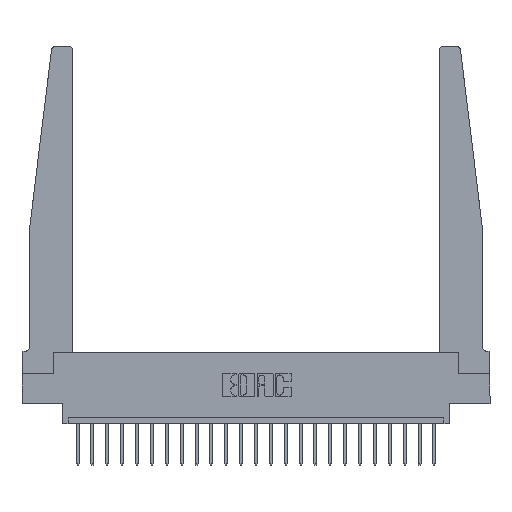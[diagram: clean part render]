
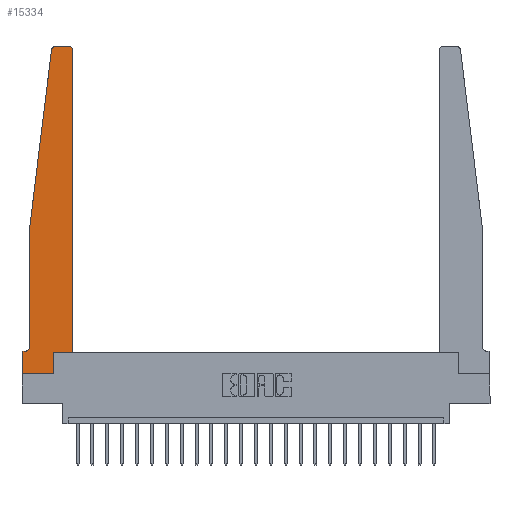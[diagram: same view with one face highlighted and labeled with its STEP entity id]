
A CAD part, top view. The second image highlights one B-rep face of the part: STEP entity #15334.
In plain terms, the highlighted planar face has unit normal (0, 0, 1).
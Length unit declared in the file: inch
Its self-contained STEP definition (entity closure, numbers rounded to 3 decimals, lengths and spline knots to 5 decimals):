
#33 = ORIENTED_EDGE ( 'NONE', *, *, #2046, .T. ) ;
#178 = VECTOR ( 'NONE', #5437, 39.37008 ) ;
#296 = EDGE_CURVE ( 'NONE', #17485, #15107, #15571, .T. ) ;
#578 = VERTEX_POINT ( 'NONE', #1605 ) ;
#906 = CARTESIAN_POINT ( 'NONE',  ( 0., 0.1875, 0.37 ) ) ;
#1040 = VECTOR ( 'NONE', #8068, 39.37008 ) ;
#1192 = CARTESIAN_POINT ( 'NONE',  ( 0.065, 1.25, 0.37 ) ) ;
#1251 = CARTESIAN_POINT ( 'NONE',  ( 0.25, 2.75, 0.37 ) ) ;
#1531 = CARTESIAN_POINT ( 'NONE',  ( 0., 0.1875, 0.37 ) ) ;
#1605 = CARTESIAN_POINT ( 'NONE',  ( 0.015, 0.1875, 0.37 ) ) ;
#2046 = EDGE_CURVE ( 'NONE', #578, #8622, #7884, .T. ) ;
#2065 = CARTESIAN_POINT ( 'NONE',  ( 0., 0., 0.37 ) ) ;
#2200 = DIRECTION ( 'NONE',  ( 1., 0., 0. ) ) ;
#2301 = CARTESIAN_POINT ( 'NONE',  ( 0.425, 0.18, 0.37 ) ) ;
#2494 = LINE ( 'NONE', #1192, #17571 ) ;
#3321 = DIRECTION ( 'NONE',  ( 1., 0., 0. ) ) ;
#3685 = LINE ( 'NONE', #8054, #11895 ) ;
#3726 = VERTEX_POINT ( 'NONE', #7447 ) ;
#3820 = ORIENTED_EDGE ( 'NONE', *, *, #14248, .T. ) ;
#4099 = EDGE_CURVE ( 'NONE', #8622, #10475, #9236, .T. ) ;
#4494 = VECTOR ( 'NONE', #9052, 39.37008 ) ;
#4500 = VECTOR ( 'NONE', #11226, 39.37008 ) ;
#5191 = DIRECTION ( 'NONE',  ( -1., 0., 0. ) ) ;
#5437 = DIRECTION ( 'NONE',  ( 1., 0., 0. ) ) ;
#5623 = LINE ( 'NONE', #1251, #7583 ) ;
#6602 = DIRECTION ( 'NONE',  ( 0., -1., 0. ) ) ;
#6870 = CARTESIAN_POINT ( 'NONE',  ( 0.27653, 2.72, 0.37 ) ) ;
#7027 = DIRECTION ( 'NONE',  ( 0., 0., 1. ) ) ;
#7152 = CIRCLE ( 'NONE', #14906, 0.03 ) ;
#7227 = AXIS2_PLACEMENT_3D ( 'NONE', #16472, #20184, #21952 ) ;
#7410 = ORIENTED_EDGE ( 'NONE', *, *, #16165, .T. ) ;
#7447 = CARTESIAN_POINT ( 'NONE',  ( 0.395, 2.75, 0.37 ) ) ;
#7566 = EDGE_CURVE ( 'NONE', #19655, #578, #7614, .T. ) ;
#7583 = VECTOR ( 'NONE', #5191, 39.37008 ) ;
#7614 = CIRCLE ( 'NONE', #7227, 0.05 ) ;
#7641 = AXIS2_PLACEMENT_3D ( 'NONE', #1531, #13812, #3321 ) ;
#7884 = LINE ( 'NONE', #9121, #17400 ) ;
#7987 = CIRCLE ( 'NONE', #13327, 0.03 ) ;
#8054 = CARTESIAN_POINT ( 'NONE',  ( 0.425, 0.18, 0.37 ) ) ;
#8068 = DIRECTION ( 'NONE',  ( -0.122, -0.992, 0. ) ) ;
#8076 = ORIENTED_EDGE ( 'NONE', *, *, #4099, .T. ) ;
#8575 = VERTEX_POINT ( 'NONE', #14924 ) ;
#8622 = VERTEX_POINT ( 'NONE', #906 ) ;
#9052 = DIRECTION ( 'NONE',  ( 0., -1., 0. ) ) ;
#9121 = CARTESIAN_POINT ( 'NONE',  ( 0.065, 0.1875, 0.37 ) ) ;
#9236 = LINE ( 'NONE', #2065, #4494 ) ;
#9386 = CARTESIAN_POINT ( 'NONE',  ( 0., 0., 0.37 ) ) ;
#9550 = CARTESIAN_POINT ( 'NONE',  ( 0.065, 0.2375, 0.37 ) ) ;
#9798 = CARTESIAN_POINT ( 'NONE',  ( 0.2605, 0.18, 0.37 ) ) ;
#9815 = CARTESIAN_POINT ( 'NONE',  ( 0.065, 1.25, 0.37 ) ) ;
#10367 = ORIENTED_EDGE ( 'NONE', *, *, #19819, .T. ) ;
#10457 = EDGE_LOOP ( 'NONE', ( #3820, #7410, #16579, #10367, #12165, #33, #8076, #15566, #21629, #22363, #20097, #19935 ) ) ;
#10475 = VERTEX_POINT ( 'NONE', #9386 ) ;
#10541 = EDGE_CURVE ( 'NONE', #21972, #19826, #13118, .T. ) ;
#10575 = CARTESIAN_POINT ( 'NONE',  ( 0., 0., 0.37 ) ) ;
#11226 = DIRECTION ( 'NONE',  ( 0., 1., 0. ) ) ;
#11419 = EDGE_CURVE ( 'NONE', #10475, #14870, #13098, .T. ) ;
#11895 = VECTOR ( 'NONE', #14939, 39.37008 ) ;
#12165 = ORIENTED_EDGE ( 'NONE', *, *, #7566, .T. ) ;
#12744 = LINE ( 'NONE', #9798, #4500 ) ;
#12791 = EDGE_CURVE ( 'NONE', #14870, #17485, #12744, .T. ) ;
#13098 = LINE ( 'NONE', #10575, #178 ) ;
#13118 = LINE ( 'NONE', #9815, #1040 ) ;
#13327 = AXIS2_PLACEMENT_3D ( 'NONE', #6870, #13493, #19040 ) ;
#13493 = DIRECTION ( 'NONE',  ( 0., 0., 1. ) ) ;
#13812 = DIRECTION ( 'NONE',  ( 0., 0., 1. ) ) ;
#14248 = EDGE_CURVE ( 'NONE', #3726, #8575, #5623, .T. ) ;
#14870 = VERTEX_POINT ( 'NONE', #20574 ) ;
#14906 = AXIS2_PLACEMENT_3D ( 'NONE', #20999, #7027, #2200 ) ;
#14922 = DIRECTION ( 'NONE',  ( -1., 0., 0. ) ) ;
#14924 = CARTESIAN_POINT ( 'NONE',  ( 0.27653, 2.75, 0.37 ) ) ;
#14939 = DIRECTION ( 'NONE',  ( 0., 1., 0. ) ) ;
#15107 = VERTEX_POINT ( 'NONE', #2301 ) ;
#15334 = ADVANCED_FACE ( 'NONE', ( #22745 ), #22539, .T. ) ;
#15566 = ORIENTED_EDGE ( 'NONE', *, *, #11419, .T. ) ;
#15571 = LINE ( 'NONE', #21371, #16116 ) ;
#16116 = VECTOR ( 'NONE', #19822, 39.37008 ) ;
#16165 = EDGE_CURVE ( 'NONE', #8575, #21972, #7987, .T. ) ;
#16240 = EDGE_CURVE ( 'NONE', #17730, #3726, #7152, .T. ) ;
#16472 = CARTESIAN_POINT ( 'NONE',  ( 0.015, 0.2375, 0.37 ) ) ;
#16579 = ORIENTED_EDGE ( 'NONE', *, *, #10541, .T. ) ;
#17033 = CARTESIAN_POINT ( 'NONE',  ( 0.065, 1.25, 0.37 ) ) ;
#17400 = VECTOR ( 'NONE', #14922, 39.37008 ) ;
#17485 = VERTEX_POINT ( 'NONE', #21920 ) ;
#17571 = VECTOR ( 'NONE', #6602, 39.37008 ) ;
#17730 = VERTEX_POINT ( 'NONE', #21278 ) ;
#19040 = DIRECTION ( 'NONE',  ( 1., 0., 0. ) ) ;
#19085 = EDGE_CURVE ( 'NONE', #15107, #17730, #3685, .T. ) ;
#19655 = VERTEX_POINT ( 'NONE', #9550 ) ;
#19819 = EDGE_CURVE ( 'NONE', #19826, #19655, #2494, .T. ) ;
#19822 = DIRECTION ( 'NONE',  ( 1., 0., 0. ) ) ;
#19826 = VERTEX_POINT ( 'NONE', #17033 ) ;
#19935 = ORIENTED_EDGE ( 'NONE', *, *, #16240, .T. ) ;
#20097 = ORIENTED_EDGE ( 'NONE', *, *, #19085, .T. ) ;
#20184 = DIRECTION ( 'NONE',  ( 0., 0., -1. ) ) ;
#20574 = CARTESIAN_POINT ( 'NONE',  ( 0.2605, 0., 0.37 ) ) ;
#20978 = CARTESIAN_POINT ( 'NONE',  ( 0.24675, 2.72367, 0.37 ) ) ;
#20999 = CARTESIAN_POINT ( 'NONE',  ( 0.395, 2.72, 0.37 ) ) ;
#21278 = CARTESIAN_POINT ( 'NONE',  ( 0.425, 2.72, 0.37 ) ) ;
#21371 = CARTESIAN_POINT ( 'NONE',  ( 0.425, 0.18, 0.37 ) ) ;
#21629 = ORIENTED_EDGE ( 'NONE', *, *, #12791, .T. ) ;
#21920 = CARTESIAN_POINT ( 'NONE',  ( 0.2605, 0.18, 0.37 ) ) ;
#21952 = DIRECTION ( 'NONE',  ( -1., 0., 0. ) ) ;
#21972 = VERTEX_POINT ( 'NONE', #20978 ) ;
#22363 = ORIENTED_EDGE ( 'NONE', *, *, #296, .T. ) ;
#22539 = PLANE ( 'NONE',  #7641 ) ;
#22745 = FACE_OUTER_BOUND ( 'NONE', #10457, .T. ) ;
